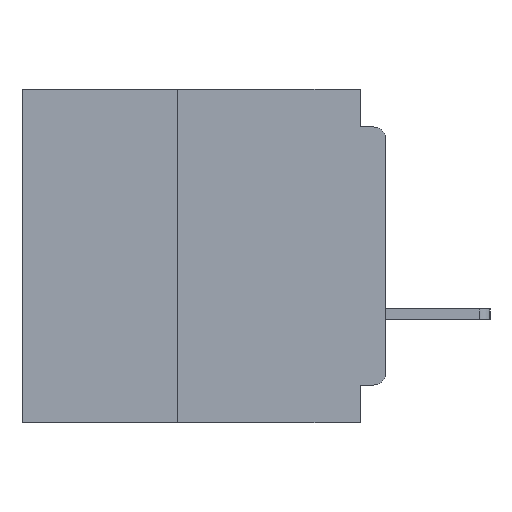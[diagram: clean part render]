
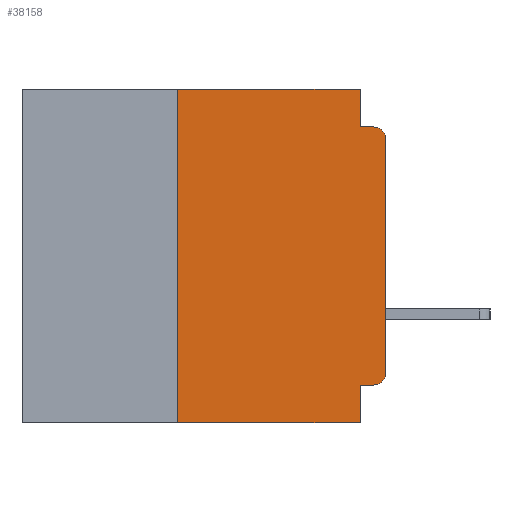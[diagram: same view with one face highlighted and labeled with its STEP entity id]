
A CAD part, left-side view. The second image highlights one B-rep face of the part: STEP entity #38158.
In plain terms, the highlighted planar face has unit normal (-1, 0, 0).
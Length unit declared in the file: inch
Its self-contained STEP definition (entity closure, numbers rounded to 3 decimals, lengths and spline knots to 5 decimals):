
#116 = VERTEX_POINT ( 'NONE', #6713 ) ;
#210 = AXIS2_PLACEMENT_3D ( 'NONE', #15278, #37527, #18464 ) ;
#233 = EDGE_CURVE ( 'NONE', #116, #11468, #19113, .T. ) ;
#588 = CIRCLE ( 'NONE', #210, 0.015 ) ;
#838 = CARTESIAN_POINT ( 'NONE',  ( 0., 0.437, 0. ) ) ;
#1149 = VECTOR ( 'NONE', #4097, 39.37008 ) ;
#1412 = LINE ( 'NONE', #5192, #16332 ) ;
#1756 = CARTESIAN_POINT ( 'NONE',  ( 0., 0.015, -0.045 ) ) ;
#1966 = LINE ( 'NONE', #22196, #17878 ) ;
#2252 = VECTOR ( 'NONE', #36369, 39.37008 ) ;
#3177 = CARTESIAN_POINT ( 'NONE',  ( 0., 0.25, 0. ) ) ;
#3269 = LINE ( 'NONE', #26704, #2252 ) ;
#3499 = CARTESIAN_POINT ( 'NONE',  ( 0., 0., -0.06 ) ) ;
#3518 = EDGE_CURVE ( 'NONE', #11468, #7220, #1966, .T. ) ;
#3798 = EDGE_CURVE ( 'NONE', #39283, #9794, #15366, .T. ) ;
#4097 = DIRECTION ( 'NONE',  ( 0., -1., 0. ) ) ;
#4396 = VERTEX_POINT ( 'NONE', #1756 ) ;
#4803 = LINE ( 'NONE', #20646, #21687 ) ;
#5192 = CARTESIAN_POINT ( 'NONE',  ( 0., 0., -0.045 ) ) ;
#6713 = CARTESIAN_POINT ( 'NONE',  ( 0., 0.015, -0.355 ) ) ;
#7138 = DIRECTION ( 'NONE',  ( 1., 0., 0. ) ) ;
#7220 = VERTEX_POINT ( 'NONE', #20636 ) ;
#7318 = LINE ( 'NONE', #34946, #14730 ) ;
#7536 = EDGE_CURVE ( 'NONE', #12824, #38371, #7318, .T. ) ;
#7933 = VECTOR ( 'NONE', #16497, 39.37008 ) ;
#9794 = VERTEX_POINT ( 'NONE', #3499 ) ;
#10416 = VERTEX_POINT ( 'NONE', #3177 ) ;
#10467 = VERTEX_POINT ( 'NONE', #16212 ) ;
#11413 = CARTESIAN_POINT ( 'NONE',  ( 0., 0.031, -0.355 ) ) ;
#11468 = VERTEX_POINT ( 'NONE', #11413 ) ;
#11965 = ORIENTED_EDGE ( 'NONE', *, *, #33941, .T. ) ;
#12555 = EDGE_LOOP ( 'NONE', ( #23534, #19746, #20443, #31940, #22283, #17224, #41228, #38118, #20351, #11965 ) ) ;
#12568 = CARTESIAN_POINT ( 'NONE',  ( 0., 0.015, -0.06 ) ) ;
#12824 = VERTEX_POINT ( 'NONE', #31710 ) ;
#12979 = EDGE_CURVE ( 'NONE', #10416, #12824, #26484, .T. ) ;
#14730 = VECTOR ( 'NONE', #19092, 39.37008 ) ;
#15278 = CARTESIAN_POINT ( 'NONE',  ( 0., 0.015, -0.34 ) ) ;
#15366 = LINE ( 'NONE', #16505, #7933 ) ;
#15789 = DIRECTION ( 'NONE',  ( 0., 0., -1. ) ) ;
#16116 = VECTOR ( 'NONE', #37362, 39.37008 ) ;
#16212 = CARTESIAN_POINT ( 'NONE',  ( 0., 0.25, -0.4 ) ) ;
#16332 = VECTOR ( 'NONE', #21130, 39.37008 ) ;
#16497 = DIRECTION ( 'NONE',  ( 0., 0., 1. ) ) ;
#16505 = CARTESIAN_POINT ( 'NONE',  ( 0., 0., 0. ) ) ;
#16565 = PLANE ( 'NONE',  #27934 ) ;
#17224 = ORIENTED_EDGE ( 'NONE', *, *, #21468, .F. ) ;
#17709 = FACE_OUTER_BOUND ( 'NONE', #12555, .T. ) ;
#17878 = VECTOR ( 'NONE', #21974, 39.37008 ) ;
#18464 = DIRECTION ( 'NONE',  ( 0., 0., -1. ) ) ;
#19092 = DIRECTION ( 'NONE',  ( 0., 0., -1. ) ) ;
#19113 = LINE ( 'NONE', #37445, #16116 ) ;
#19446 = EDGE_CURVE ( 'NONE', #38371, #4396, #1412, .T. ) ;
#19746 = ORIENTED_EDGE ( 'NONE', *, *, #40718, .T. ) ;
#20351 = ORIENTED_EDGE ( 'NONE', *, *, #233, .F. ) ;
#20443 = ORIENTED_EDGE ( 'NONE', *, *, #19446, .F. ) ;
#20636 = CARTESIAN_POINT ( 'NONE',  ( 0., 0.031, -0.4 ) ) ;
#20646 = CARTESIAN_POINT ( 'NONE',  ( 0., 0.25, -0.4 ) ) ;
#21130 = DIRECTION ( 'NONE',  ( 0., -1., 0. ) ) ;
#21468 = EDGE_CURVE ( 'NONE', #10467, #10416, #4803, .T. ) ;
#21687 = VECTOR ( 'NONE', #33424, 39.37008 ) ;
#21974 = DIRECTION ( 'NONE',  ( 0., 0., -1. ) ) ;
#22196 = CARTESIAN_POINT ( 'NONE',  ( 0., 0.031, -0.4 ) ) ;
#22283 = ORIENTED_EDGE ( 'NONE', *, *, #12979, .F. ) ;
#23534 = ORIENTED_EDGE ( 'NONE', *, *, #3798, .T. ) ;
#23720 = CARTESIAN_POINT ( 'NONE',  ( 0., 0.031, -0.045 ) ) ;
#25418 = CIRCLE ( 'NONE', #37917, 0.015 ) ;
#26088 = CARTESIAN_POINT ( 'NONE',  ( 0., 0.437, 0. ) ) ;
#26484 = LINE ( 'NONE', #838, #1149 ) ;
#26704 = CARTESIAN_POINT ( 'NONE',  ( 0., 0.437, -0.4 ) ) ;
#27934 = AXIS2_PLACEMENT_3D ( 'NONE', #26088, #7138, #29311 ) ;
#28409 = EDGE_CURVE ( 'NONE', #10467, #7220, #3269, .T. ) ;
#29311 = DIRECTION ( 'NONE',  ( 0., 0., -1. ) ) ;
#31710 = CARTESIAN_POINT ( 'NONE',  ( 0., 0.031, 0. ) ) ;
#31940 = ORIENTED_EDGE ( 'NONE', *, *, #7536, .F. ) ;
#33424 = DIRECTION ( 'NONE',  ( 0., 0., 1. ) ) ;
#33941 = EDGE_CURVE ( 'NONE', #116, #39283, #588, .T. ) ;
#34840 = DIRECTION ( 'NONE',  ( -1., 0., 0. ) ) ;
#34946 = CARTESIAN_POINT ( 'NONE',  ( 0., 0.031, 0. ) ) ;
#36369 = DIRECTION ( 'NONE',  ( 0., -1., 0. ) ) ;
#37362 = DIRECTION ( 'NONE',  ( 0., 1., 0. ) ) ;
#37445 = CARTESIAN_POINT ( 'NONE',  ( 0., 0., -0.355 ) ) ;
#37527 = DIRECTION ( 'NONE',  ( -1., 0., 0. ) ) ;
#37917 = AXIS2_PLACEMENT_3D ( 'NONE', #12568, #34840, #15789 ) ;
#38118 = ORIENTED_EDGE ( 'NONE', *, *, #3518, .F. ) ;
#38158 = ADVANCED_FACE ( 'NONE', ( #17709 ), #16565, .F. ) ;
#38316 = CARTESIAN_POINT ( 'NONE',  ( 0., 0., -0.34 ) ) ;
#38371 = VERTEX_POINT ( 'NONE', #23720 ) ;
#39283 = VERTEX_POINT ( 'NONE', #38316 ) ;
#40718 = EDGE_CURVE ( 'NONE', #9794, #4396, #25418, .T. ) ;
#41228 = ORIENTED_EDGE ( 'NONE', *, *, #28409, .T. ) ;
